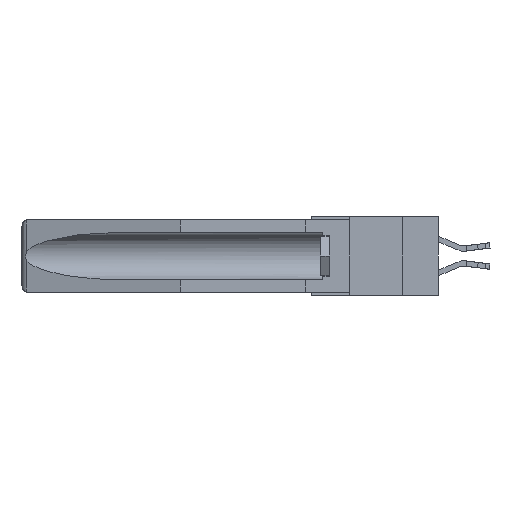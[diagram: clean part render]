
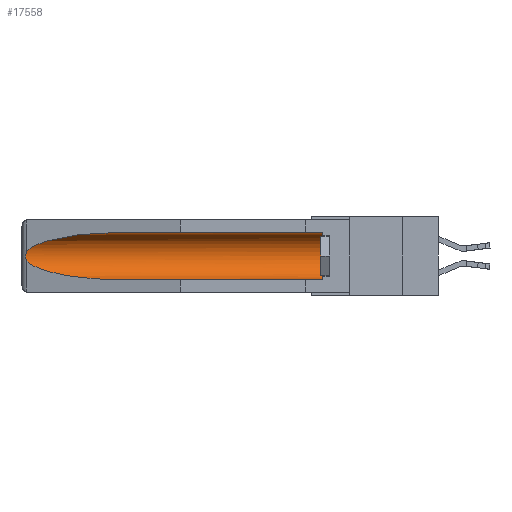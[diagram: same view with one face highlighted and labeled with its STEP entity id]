
A CAD part, left-side view. The second image highlights one B-rep face of the part: STEP entity #17558.
In plain terms, the highlighted cylindrical face has radius 2.857 mm (diameter 5.715 mm), a partial arc.
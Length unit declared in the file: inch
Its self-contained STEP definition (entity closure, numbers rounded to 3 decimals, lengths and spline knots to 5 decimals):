
#291 = CARTESIAN_POINT ( 'NONE',  ( 0.26537, 1.52718, -0.14972 ) ) ;
#893 = CIRCLE ( 'NONE', #10170, 0.1125 ) ;
#1542 = CARTESIAN_POINT ( 'NONE',  ( 0.26597, 1.52961, -0.15275 ) ) ;
#1774 = VERTEX_POINT ( 'NONE', #13284 ) ;
#1867 = CARTESIAN_POINT ( 'NONE',  ( 0.26597, 1.5296, -0.19026 ) ) ;
#2092 = VECTOR ( 'NONE', #25155, 39.37008 ) ;
#2268 = CARTESIAN_POINT ( 'NONE',  ( 0.155, 0.126, -0.1715 ) ) ;
#2370 = VERTEX_POINT ( 'NONE', #18576 ) ;
#2937 = VERTEX_POINT ( 'NONE', #16973 ) ;
#3066 = CARTESIAN_POINT ( 'NONE',  ( 0.21114, 1.30732, -0.059 ) ) ;
#3436 = ORIENTED_EDGE ( 'NONE', *, *, #4431, .T. ) ;
#3855 = CARTESIAN_POINT ( 'NONE',  ( 0.155, 1.07973, -0.284 ) ) ;
#3859 = CARTESIAN_POINT ( 'NONE',  ( 0.2675, 1.53308, -0.17534 ) ) ;
#4175 = ORIENTED_EDGE ( 'NONE', *, *, #15888, .T. ) ;
#4288 = VECTOR ( 'NONE', #5718, 39.37008 ) ;
#4431 = EDGE_CURVE ( 'NONE', #1774, #13148, #25711, .T. ) ;
#4443 = DIRECTION ( 'NONE',  ( 0., 1., 0. ) ) ;
#4602 = B_SPLINE_CURVE_WITH_KNOTS ( 'NONE', 3,
 ( #7539, #1542, #24287, #16379, #18106, #3859, #12249, #5814, #1867, #6070 ),
 .UNSPECIFIED., .F., .F.,
 ( 4, 2, 2, 2, 4 ),
 ( 0., 0.00029, 0.00058, 0.00087, 0.00117 ),
 .UNSPECIFIED. ) ;
#5718 = DIRECTION ( 'NONE',  ( 0., 1., 0. ) ) ;
#5814 = CARTESIAN_POINT ( 'NONE',  ( 0.26655, 1.53094, -0.18657 ) ) ;
#6070 = CARTESIAN_POINT ( 'NONE',  ( 0.26537, 1.52718, -0.19328 ) ) ;
#6385 = DIRECTION ( 'NONE',  ( 0., -1., 0. ) ) ;
#7539 = CARTESIAN_POINT ( 'NONE',  ( 0.26537, 1.52718, -0.14972 ) ) ;
#7718 = CARTESIAN_POINT ( 'NONE',  ( 0.26537, 1.52718, -0.19328 ) ) ;
#9543 = CARTESIAN_POINT ( 'NONE',  ( 0.155, 1.07973, -0.284 ) ) ;
#9740 = LINE ( 'NONE', #13863, #4288 ) ;
#10170 = AXIS2_PLACEMENT_3D ( 'NONE', #2268, #6385, #18575 ) ;
#10274 = ORIENTED_EDGE ( 'NONE', *, *, #18986, .T. ) ;
#10781 = ORIENTED_EDGE ( 'NONE', *, *, #17161, .T. ) ;
#11911 = CARTESIAN_POINT ( 'NONE',  ( 0.25451, 1.48313, -0.24835 ) ) ;
#12249 = CARTESIAN_POINT ( 'NONE',  ( 0.2673, 1.53269, -0.17917 ) ) ;
#12684 = DIRECTION ( 'NONE',  ( 0., 0., 1. ) ) ;
#13148 = VERTEX_POINT ( 'NONE', #291 ) ;
#13284 = CARTESIAN_POINT ( 'NONE',  ( 0.155, 1.07973, -0.059 ) ) ;
#13290 = CARTESIAN_POINT ( 'NONE',  ( 0.26537, 1.52718, -0.14972 ) ) ;
#13863 = CARTESIAN_POINT ( 'NONE',  ( 0.155, -0.30754, -0.284 ) ) ;
#14555 = VERTEX_POINT ( 'NONE', #19156 ) ;
#14986 =( BOUNDED_CURVE ( )  B_SPLINE_CURVE ( 3, ( #7718, #11911, #15948, #3855 ),
 .UNSPECIFIED., .F., .F. ) 
 B_SPLINE_CURVE_WITH_KNOTS ( ( 4, 4 ),
 ( 0.1948, 1.5708 ),
 .UNSPECIFIED. ) 
 CURVE ( )  GEOMETRIC_REPRESENTATION_ITEM ( )  RATIONAL_B_SPLINE_CURVE ( ( 1., 0.848, 0.848, 1. ) ) 
 REPRESENTATION_ITEM ( '' )  );
#15265 = LINE ( 'NONE', #22857, #2092 ) ;
#15888 = EDGE_CURVE ( 'NONE', #2370, #1774, #15265, .T. ) ;
#15948 = CARTESIAN_POINT ( 'NONE',  ( 0.21114, 1.30732, -0.284 ) ) ;
#16379 = CARTESIAN_POINT ( 'NONE',  ( 0.2673, 1.5327, -0.16383 ) ) ;
#16608 = ORIENTED_EDGE ( 'NONE', *, *, #24609, .T. ) ;
#16728 = CARTESIAN_POINT ( 'NONE',  ( 0.155, -0.30754, -0.1715 ) ) ;
#16973 = CARTESIAN_POINT ( 'NONE',  ( 0.155, 0.126, -0.284 ) ) ;
#17148 = CARTESIAN_POINT ( 'NONE',  ( 0.155, 1.07973, -0.059 ) ) ;
#17161 = EDGE_CURVE ( 'NONE', #13148, #14555, #4602, .T. ) ;
#17558 = ADVANCED_FACE ( 'NONE', ( #26286 ), #24368, .F. ) ;
#18106 = CARTESIAN_POINT ( 'NONE',  ( 0.2675, 1.53308, -0.16763 ) ) ;
#18384 = ORIENTED_EDGE ( 'NONE', *, *, #25979, .F. ) ;
#18575 = DIRECTION ( 'NONE',  ( 0., 0., 1. ) ) ;
#18576 = CARTESIAN_POINT ( 'NONE',  ( 0.155, 0.126, -0.059 ) ) ;
#18986 = EDGE_CURVE ( 'NONE', #14555, #21581, #14986, .T. ) ;
#19101 = CARTESIAN_POINT ( 'NONE',  ( 0.25451, 1.48313, -0.09465 ) ) ;
#19156 = CARTESIAN_POINT ( 'NONE',  ( 0.26537, 1.52718, -0.19328 ) ) ;
#21513 = EDGE_LOOP ( 'NONE', ( #3436, #10781, #10274, #18384, #16608, #4175 ) ) ;
#21581 = VERTEX_POINT ( 'NONE', #9543 ) ;
#22857 = CARTESIAN_POINT ( 'NONE',  ( 0.155, -0.30754, -0.059 ) ) ;
#23723 = AXIS2_PLACEMENT_3D ( 'NONE', #16728, #4443, #12684 ) ;
#24287 = CARTESIAN_POINT ( 'NONE',  ( 0.26654, 1.53092, -0.15636 ) ) ;
#24368 = CYLINDRICAL_SURFACE ( 'NONE', #23723, 0.1125 ) ;
#24609 = EDGE_CURVE ( 'NONE', #2937, #2370, #893, .T. ) ;
#25155 = DIRECTION ( 'NONE',  ( 0., 1., 0. ) ) ;
#25711 =( BOUNDED_CURVE ( )  B_SPLINE_CURVE ( 3, ( #17148, #3066, #19101, #13290 ),
 .UNSPECIFIED., .F., .F. ) 
 B_SPLINE_CURVE_WITH_KNOTS ( ( 4, 4 ),
 ( 4.71239, 6.08839 ),
 .UNSPECIFIED. ) 
 CURVE ( )  GEOMETRIC_REPRESENTATION_ITEM ( )  RATIONAL_B_SPLINE_CURVE ( ( 1., 0.848, 0.848, 1. ) ) 
 REPRESENTATION_ITEM ( '' )  );
#25979 = EDGE_CURVE ( 'NONE', #2937, #21581, #9740, .T. ) ;
#26286 = FACE_OUTER_BOUND ( 'NONE', #21513, .T. ) ;
